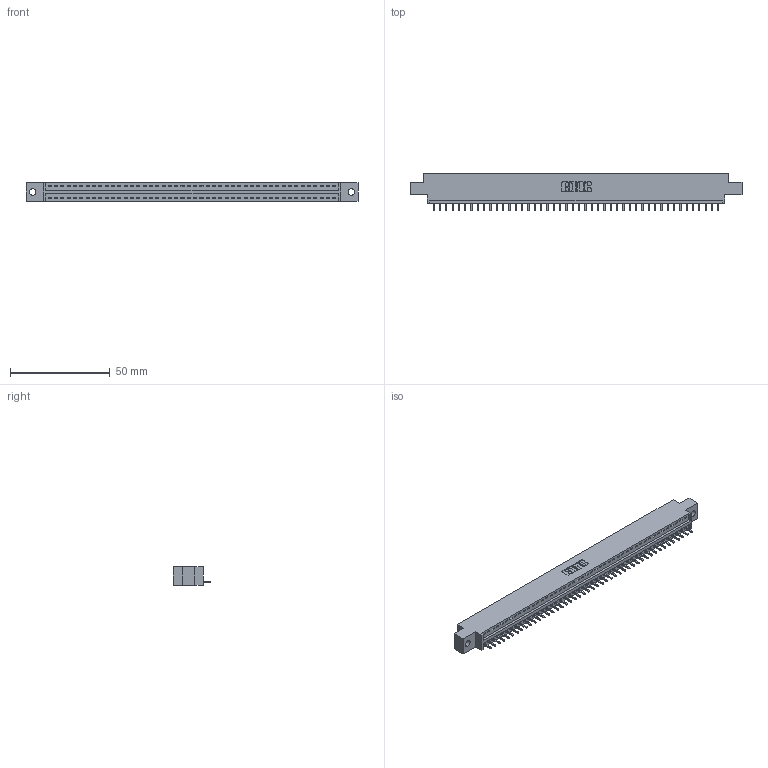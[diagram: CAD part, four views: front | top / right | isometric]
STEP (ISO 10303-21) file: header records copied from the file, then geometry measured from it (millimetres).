
FILE_DESCRIPTION (( 'STEP AP203' ), '1' );
FILE_NAME ('396-046-521-602.STEP', '2019-10-28T03:11:28', ( '' ), ( '' ), 'SwSTEP 2.0', 'SolidWorks 2016', '' );
FILE_SCHEMA (( 'CONFIG_CONTROL_DESIGN' ));
Length unit declared in the file: inch
Products named in the file (3): 346 Part_0.170 Offset - 0.128 Dia; 396-046-521-602; 345-292-001_345-293-121
Assembly tree (47 placements, depth 2):
  396-046-521-602
    346 Part_0.170 Offset - 0.128 Dia
    345-292-001_345-293-121  x46
Bounding box: 166.62 x 19.05 x 9.4 mm (x, y, z)
Volume: 15655 mm3; surface area: 18978.4 mm2
Topology: 47 solids, 47 shells, 2794 faces, 8437 edges, 5562 vertices
Faces by surface type: plane 1920, cylinder 874
Entity records: 28163 total; most frequent: CARTESIAN_POINT 4834, ORIENTED_EDGE 4814, DIRECTION 4259, EDGE_CURVE 2407, VECTOR 2091, LINE 2091, VERTEX_POINT 1602, AXIS2_PLACEMENT_3D 1084
